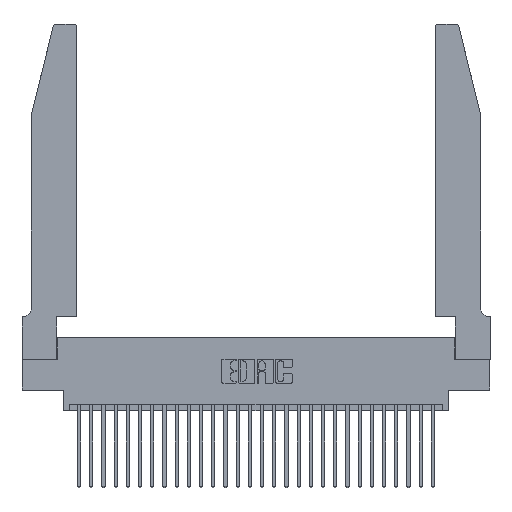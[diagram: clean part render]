
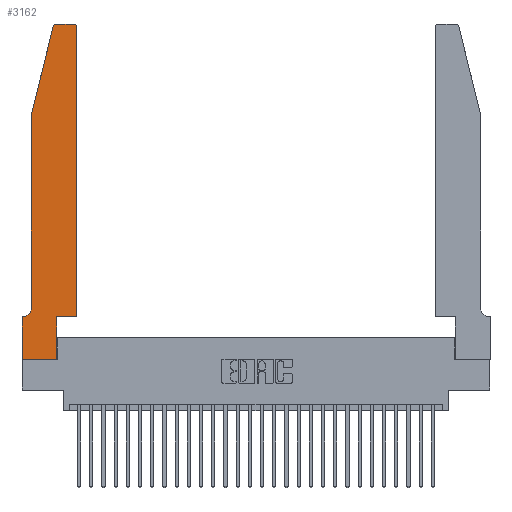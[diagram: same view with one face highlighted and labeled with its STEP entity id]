
A CAD part, top view. The second image highlights one B-rep face of the part: STEP entity #3162.
In plain terms, the highlighted planar face has unit normal (0, 0, 1).
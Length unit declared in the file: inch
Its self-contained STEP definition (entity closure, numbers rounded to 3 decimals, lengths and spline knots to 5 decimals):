
#359 = EDGE_CURVE ( 'NONE', #9370, #18614, #27078, .T. ) ;
#583 = ORIENTED_EDGE ( 'NONE', *, *, #27652, .T. ) ;
#652 = VERTEX_POINT ( 'NONE', #3375 ) ;
#903 = ORIENTED_EDGE ( 'NONE', *, *, #4908, .T. ) ;
#1164 = DIRECTION ( 'NONE',  ( 0., 0., -1. ) ) ;
#1993 = EDGE_CURVE ( 'NONE', #15611, #9017, #15210, .T. ) ;
#2172 = CIRCLE ( 'NONE', #10267, 0.03 ) ;
#3162 = ADVANCED_FACE ( 'NONE', ( #21121 ), #9303, .T. ) ;
#3375 = CARTESIAN_POINT ( 'NONE',  ( 0.4505, 2.72, 0.37 ) ) ;
#3454 = VECTOR ( 'NONE', #12128, 39.37008 ) ;
#3557 = VERTEX_POINT ( 'NONE', #15538 ) ;
#3818 = CARTESIAN_POINT ( 'NONE',  ( 0.0755, 2., 0.37 ) ) ;
#3922 = ORIENTED_EDGE ( 'NONE', *, *, #15164, .T. ) ;
#3928 = CARTESIAN_POINT ( 'NONE',  ( 0.2865, 0., 0.37 ) ) ;
#4198 = LINE ( 'NONE', #16796, #3454 ) ;
#4908 = EDGE_CURVE ( 'NONE', #20047, #652, #22070, .T. ) ;
#5386 = ORIENTED_EDGE ( 'NONE', *, *, #20946, .T. ) ;
#5990 = CARTESIAN_POINT ( 'NONE',  ( 0., 0.35, 0.37 ) ) ;
#6127 = ORIENTED_EDGE ( 'NONE', *, *, #16883, .T. ) ;
#6144 = ORIENTED_EDGE ( 'NONE', *, *, #25640, .T. ) ;
#6401 = VECTOR ( 'NONE', #29285, 39.37008 ) ;
#6527 = VERTEX_POINT ( 'NONE', #20955 ) ;
#6669 = CIRCLE ( 'NONE', #22677, 0.03 ) ;
#6705 = VERTEX_POINT ( 'NONE', #16878 ) ;
#6917 = DIRECTION ( 'NONE',  ( 0., 1., 0. ) ) ;
#6967 = LINE ( 'NONE', #18355, #19378 ) ;
#7246 = ORIENTED_EDGE ( 'NONE', *, *, #28849, .T. ) ;
#7447 = AXIS2_PLACEMENT_3D ( 'NONE', #29904, #27714, #14072 ) ;
#8415 = DIRECTION ( 'NONE',  ( -1., 0., 0. ) ) ;
#8425 = EDGE_CURVE ( 'NONE', #6705, #15958, #6967, .T. ) ;
#8532 = CARTESIAN_POINT ( 'NONE',  ( 0.4505, 0.35, 0.37 ) ) ;
#8879 = VECTOR ( 'NONE', #25829, 39.37008 ) ;
#9017 = VERTEX_POINT ( 'NONE', #29781 ) ;
#9303 = PLANE ( 'NONE',  #7447 ) ;
#9370 = VERTEX_POINT ( 'NONE', #20771 ) ;
#9712 = CARTESIAN_POINT ( 'NONE',  ( 0.2865, 0.35, 0.37 ) ) ;
#9845 = ORIENTED_EDGE ( 'NONE', *, *, #359, .T. ) ;
#10267 = AXIS2_PLACEMENT_3D ( 'NONE', #24759, #10994, #27062 ) ;
#10994 = DIRECTION ( 'NONE',  ( 0., 0., 1. ) ) ;
#11701 = AXIS2_PLACEMENT_3D ( 'NONE', #15363, #1164, #17666 ) ;
#12128 = DIRECTION ( 'NONE',  ( 0., -1., 0. ) ) ;
#12362 = VECTOR ( 'NONE', #24771, 39.37008 ) ;
#12640 = DIRECTION ( 'NONE',  ( 0., 0., 1. ) ) ;
#12788 = ORIENTED_EDGE ( 'NONE', *, *, #8425, .T. ) ;
#13329 = CARTESIAN_POINT ( 'NONE',  ( 0.0755, 2., 0.37 ) ) ;
#13767 = DIRECTION ( 'NONE',  ( 1., 0., 0. ) ) ;
#14072 = DIRECTION ( 'NONE',  ( 1., 0., 0. ) ) ;
#14615 = VECTOR ( 'NONE', #6917, 39.37008 ) ;
#15164 = EDGE_CURVE ( 'NONE', #6527, #9370, #28262, .T. ) ;
#15210 = LINE ( 'NONE', #20453, #27332 ) ;
#15363 = CARTESIAN_POINT ( 'NONE',  ( 0.0055, 0.42, 0.37 ) ) ;
#15538 = CARTESIAN_POINT ( 'NONE',  ( 0.0755, 2., 0.37 ) ) ;
#15596 = EDGE_CURVE ( 'NONE', #28220, #20047, #16295, .T. ) ;
#15611 = VERTEX_POINT ( 'NONE', #21523 ) ;
#15958 = VERTEX_POINT ( 'NONE', #3928 ) ;
#16295 = LINE ( 'NONE', #21324, #21660 ) ;
#16408 = ORIENTED_EDGE ( 'NONE', *, *, #17276, .T. ) ;
#16796 = CARTESIAN_POINT ( 'NONE',  ( 0., 0., 0.37 ) ) ;
#16878 = CARTESIAN_POINT ( 'NONE',  ( 0., 0., 0.37 ) ) ;
#16883 = EDGE_CURVE ( 'NONE', #652, #15611, #6669, .T. ) ;
#17276 = EDGE_CURVE ( 'NONE', #15958, #28220, #21211, .T. ) ;
#17666 = DIRECTION ( 'NONE',  ( -1., 0., 0. ) ) ;
#18355 = CARTESIAN_POINT ( 'NONE',  ( 0., 0., 0.37 ) ) ;
#18478 = LINE ( 'NONE', #3818, #12362 ) ;
#18614 = VERTEX_POINT ( 'NONE', #5990 ) ;
#19378 = VECTOR ( 'NONE', #13767, 39.37008 ) ;
#19823 = DIRECTION ( 'NONE',  ( -1., 0., 0. ) ) ;
#20047 = VERTEX_POINT ( 'NONE', #8532 ) ;
#20453 = CARTESIAN_POINT ( 'NONE',  ( 0.2605, 2.75, 0.37 ) ) ;
#20771 = CARTESIAN_POINT ( 'NONE',  ( 0.0055, 0.35, 0.37 ) ) ;
#20946 = EDGE_CURVE ( 'NONE', #18614, #6705, #4198, .T. ) ;
#20955 = CARTESIAN_POINT ( 'NONE',  ( 0.0755, 0.42, 0.37 ) ) ;
#21121 = FACE_OUTER_BOUND ( 'NONE', #29979, .T. ) ;
#21211 = LINE ( 'NONE', #9712, #8879 ) ;
#21324 = CARTESIAN_POINT ( 'NONE',  ( 0.4505, 0.35, 0.37 ) ) ;
#21523 = CARTESIAN_POINT ( 'NONE',  ( 0.4205, 2.75, 0.37 ) ) ;
#21660 = VECTOR ( 'NONE', #26020, 39.37008 ) ;
#22012 = CARTESIAN_POINT ( 'NONE',  ( 0.25487, 2.72718, 0.37 ) ) ;
#22018 = CARTESIAN_POINT ( 'NONE',  ( 0.2865, 0.35, 0.37 ) ) ;
#22070 = LINE ( 'NONE', #25439, #14615 ) ;
#22677 = AXIS2_PLACEMENT_3D ( 'NONE', #26338, #12640, #28626 ) ;
#22867 = VERTEX_POINT ( 'NONE', #22012 ) ;
#22996 = ORIENTED_EDGE ( 'NONE', *, *, #1993, .T. ) ;
#24372 = CARTESIAN_POINT ( 'NONE',  ( 0.0755, 0.35, 0.37 ) ) ;
#24759 = CARTESIAN_POINT ( 'NONE',  ( 0.284, 2.72, 0.37 ) ) ;
#24771 = DIRECTION ( 'NONE',  ( 0., -1., 0. ) ) ;
#24884 = LINE ( 'NONE', #13329, #6401 ) ;
#25439 = CARTESIAN_POINT ( 'NONE',  ( 0.4505, 0.35, 0.37 ) ) ;
#25640 = EDGE_CURVE ( 'NONE', #3557, #6527, #18478, .T. ) ;
#25829 = DIRECTION ( 'NONE',  ( 0., 1., 0. ) ) ;
#26020 = DIRECTION ( 'NONE',  ( 1., 0., 0. ) ) ;
#26338 = CARTESIAN_POINT ( 'NONE',  ( 0.4205, 2.72, 0.37 ) ) ;
#27062 = DIRECTION ( 'NONE',  ( 1., 0., 0. ) ) ;
#27078 = LINE ( 'NONE', #24372, #27786 ) ;
#27332 = VECTOR ( 'NONE', #19823, 39.37008 ) ;
#27652 = EDGE_CURVE ( 'NONE', #9017, #22867, #2172, .T. ) ;
#27714 = DIRECTION ( 'NONE',  ( 0., 0., 1. ) ) ;
#27786 = VECTOR ( 'NONE', #8415, 39.37008 ) ;
#28220 = VERTEX_POINT ( 'NONE', #22018 ) ;
#28262 = CIRCLE ( 'NONE', #11701, 0.07 ) ;
#28626 = DIRECTION ( 'NONE',  ( 1., 0., 0. ) ) ;
#28849 = EDGE_CURVE ( 'NONE', #22867, #3557, #24884, .T. ) ;
#28891 = ORIENTED_EDGE ( 'NONE', *, *, #15596, .T. ) ;
#29285 = DIRECTION ( 'NONE',  ( -0.239, -0.971, 0. ) ) ;
#29781 = CARTESIAN_POINT ( 'NONE',  ( 0.284, 2.75, 0.37 ) ) ;
#29904 = CARTESIAN_POINT ( 'NONE',  ( 0., 0.35, 0.37 ) ) ;
#29979 = EDGE_LOOP ( 'NONE', ( #22996, #583, #7246, #6144, #3922, #9845, #5386, #12788, #16408, #28891, #903, #6127 ) ) ;
